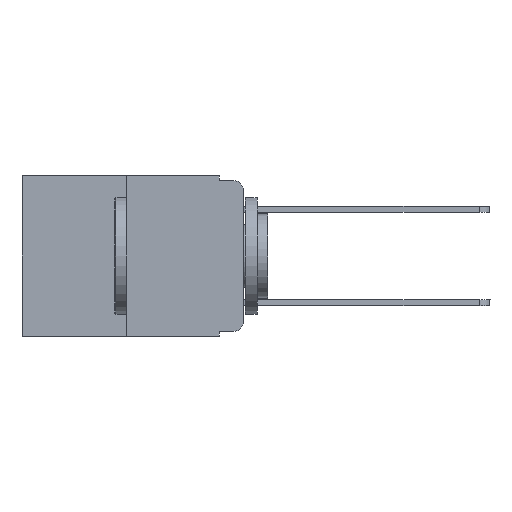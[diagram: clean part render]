
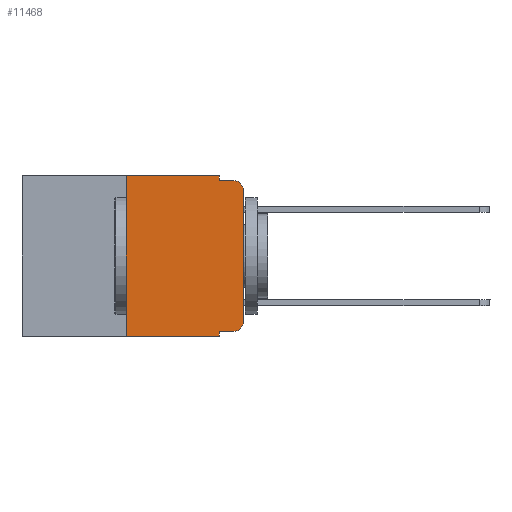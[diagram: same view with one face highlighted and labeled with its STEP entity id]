
A CAD part, left-side view. The second image highlights one B-rep face of the part: STEP entity #11468.
In plain terms, the highlighted planar face has unit normal (-1, 0, 0).
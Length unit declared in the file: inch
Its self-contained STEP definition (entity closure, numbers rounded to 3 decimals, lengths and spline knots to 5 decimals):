
#37 = EDGE_CURVE ( 'NONE', #13119, #14089, #9833, .T. ) ;
#47 = CARTESIAN_POINT ( 'NONE',  ( 0., 0.25, 0. ) ) ;
#218 = VERTEX_POINT ( 'NONE', #13717 ) ;
#460 = VECTOR ( 'NONE', #13945, 39.37008 ) ;
#554 = CARTESIAN_POINT ( 'NONE',  ( 0., 0.02, -0.313 ) ) ;
#1793 = VERTEX_POINT ( 'NONE', #3005 ) ;
#2212 = CARTESIAN_POINT ( 'NONE',  ( 0., 0.473, 0. ) ) ;
#2262 = LINE ( 'NONE', #14230, #3642 ) ;
#2435 = EDGE_CURVE ( 'NONE', #218, #8807, #7947, .T. ) ;
#2461 = DIRECTION ( 'NONE',  ( 0., -1., 0. ) ) ;
#2710 = VERTEX_POINT ( 'NONE', #14730 ) ;
#2769 = LINE ( 'NONE', #14355, #15031 ) ;
#3004 = CARTESIAN_POINT ( 'NONE',  ( 0., 0.02, -0.03 ) ) ;
#3005 = CARTESIAN_POINT ( 'NONE',  ( 0., 0.02, -0.333 ) ) ;
#3642 = VECTOR ( 'NONE', #4441, 39.37008 ) ;
#3922 = ORIENTED_EDGE ( 'NONE', *, *, #5202, .F. ) ;
#4358 = CARTESIAN_POINT ( 'NONE',  ( 0., 0.051, -0.333 ) ) ;
#4441 = DIRECTION ( 'NONE',  ( 0., 0., 1. ) ) ;
#4509 = EDGE_CURVE ( 'NONE', #2710, #1793, #15010, .T. ) ;
#4860 = CARTESIAN_POINT ( 'NONE',  ( 0., 0.051, 0. ) ) ;
#5202 = EDGE_CURVE ( 'NONE', #13119, #15027, #10749, .T. ) ;
#5244 = EDGE_CURVE ( 'NONE', #2710, #14089, #7382, .T. ) ;
#5310 = ORIENTED_EDGE ( 'NONE', *, *, #5244, .F. ) ;
#5454 = CIRCLE ( 'NONE', #13941, 0.02 ) ;
#5488 = DIRECTION ( 'NONE',  ( 0., -1., 0. ) ) ;
#5547 = EDGE_CURVE ( 'NONE', #8198, #8122, #2262, .T. ) ;
#5572 = ORIENTED_EDGE ( 'NONE', *, *, #7688, .T. ) ;
#5823 = DIRECTION ( 'NONE',  ( 0., 0., -1. ) ) ;
#5909 = ORIENTED_EDGE ( 'NONE', *, *, #12855, .F. ) ;
#5998 = CARTESIAN_POINT ( 'NONE',  ( 0., 0.02, -0.01 ) ) ;
#6306 = CARTESIAN_POINT ( 'NONE',  ( 0., 0.473, -0.343 ) ) ;
#6315 = VECTOR ( 'NONE', #5488, 39.37008 ) ;
#6698 = EDGE_LOOP ( 'NONE', ( #8453, #5572, #15199, #14697, #5909, #3922, #14849, #5310, #14864, #13732 ) ) ;
#7089 = VECTOR ( 'NONE', #9001, 39.37008 ) ;
#7211 = CARTESIAN_POINT ( 'NONE',  ( 0., 0.051, -0.01 ) ) ;
#7294 = EDGE_CURVE ( 'NONE', #1793, #8198, #5454, .T. ) ;
#7382 = LINE ( 'NONE', #4860, #12680 ) ;
#7572 = CARTESIAN_POINT ( 'NONE',  ( 0., 0.051, -0.343 ) ) ;
#7575 = VECTOR ( 'NONE', #2461, 39.37008 ) ;
#7688 = EDGE_CURVE ( 'NONE', #8122, #7881, #10988, .T. ) ;
#7785 = CARTESIAN_POINT ( 'NONE',  ( 0., 0.051, -0.01 ) ) ;
#7881 = VERTEX_POINT ( 'NONE', #5998 ) ;
#7947 = LINE ( 'NONE', #10364, #13610 ) ;
#8122 = VERTEX_POINT ( 'NONE', #11326 ) ;
#8198 = VERTEX_POINT ( 'NONE', #15049 ) ;
#8433 = DIRECTION ( 'NONE',  ( 0., -1., 0. ) ) ;
#8453 = ORIENTED_EDGE ( 'NONE', *, *, #5547, .T. ) ;
#8807 = VERTEX_POINT ( 'NONE', #7211 ) ;
#9001 = DIRECTION ( 'NONE',  ( 0., -1., 0. ) ) ;
#9741 = FACE_OUTER_BOUND ( 'NONE', #6698, .T. ) ;
#9806 = CARTESIAN_POINT ( 'NONE',  ( 0., 0.25, 0. ) ) ;
#9833 = LINE ( 'NONE', #6306, #7575 ) ;
#10364 = CARTESIAN_POINT ( 'NONE',  ( 0., 0.051, 0. ) ) ;
#10438 = DIRECTION ( 'NONE',  ( 0., 0., -1. ) ) ;
#10715 = AXIS2_PLACEMENT_3D ( 'NONE', #3004, #13586, #12426 ) ;
#10749 = LINE ( 'NONE', #47, #460 ) ;
#10988 = CIRCLE ( 'NONE', #10715, 0.02 ) ;
#11326 = CARTESIAN_POINT ( 'NONE',  ( 0., 0., -0.03 ) ) ;
#11468 = ADVANCED_FACE ( 'NONE', ( #9741 ), #14492, .F. ) ;
#11777 = DIRECTION ( 'NONE',  ( 1., 0., 0. ) ) ;
#11840 = CARTESIAN_POINT ( 'NONE',  ( 0., 0.25, -0.343 ) ) ;
#12001 = DIRECTION ( 'NONE',  ( 0., 0., -1. ) ) ;
#12426 = DIRECTION ( 'NONE',  ( 0., 0., -1. ) ) ;
#12680 = VECTOR ( 'NONE', #12001, 39.37008 ) ;
#12855 = EDGE_CURVE ( 'NONE', #15027, #218, #2769, .T. ) ;
#13119 = VERTEX_POINT ( 'NONE', #11840 ) ;
#13384 = EDGE_CURVE ( 'NONE', #8807, #7881, #13789, .T. ) ;
#13586 = DIRECTION ( 'NONE',  ( -1., 0., 0. ) ) ;
#13610 = VECTOR ( 'NONE', #10438, 39.37008 ) ;
#13717 = CARTESIAN_POINT ( 'NONE',  ( 0., 0.051, 0. ) ) ;
#13732 = ORIENTED_EDGE ( 'NONE', *, *, #7294, .T. ) ;
#13789 = LINE ( 'NONE', #7785, #6315 ) ;
#13910 = DIRECTION ( 'NONE',  ( 0., 0., -1. ) ) ;
#13941 = AXIS2_PLACEMENT_3D ( 'NONE', #554, #15148, #13910 ) ;
#13945 = DIRECTION ( 'NONE',  ( 0., 0., 1. ) ) ;
#14089 = VERTEX_POINT ( 'NONE', #7572 ) ;
#14230 = CARTESIAN_POINT ( 'NONE',  ( 0., 0., 0. ) ) ;
#14283 = AXIS2_PLACEMENT_3D ( 'NONE', #2212, #11777, #5823 ) ;
#14355 = CARTESIAN_POINT ( 'NONE',  ( 0., 0.473, 0. ) ) ;
#14492 = PLANE ( 'NONE',  #14283 ) ;
#14697 = ORIENTED_EDGE ( 'NONE', *, *, #2435, .F. ) ;
#14730 = CARTESIAN_POINT ( 'NONE',  ( 0., 0.051, -0.333 ) ) ;
#14849 = ORIENTED_EDGE ( 'NONE', *, *, #37, .T. ) ;
#14864 = ORIENTED_EDGE ( 'NONE', *, *, #4509, .T. ) ;
#15010 = LINE ( 'NONE', #4358, #7089 ) ;
#15027 = VERTEX_POINT ( 'NONE', #9806 ) ;
#15031 = VECTOR ( 'NONE', #8433, 39.37008 ) ;
#15049 = CARTESIAN_POINT ( 'NONE',  ( 0., 0., -0.313 ) ) ;
#15148 = DIRECTION ( 'NONE',  ( -1., 0., 0. ) ) ;
#15199 = ORIENTED_EDGE ( 'NONE', *, *, #13384, .F. ) ;
